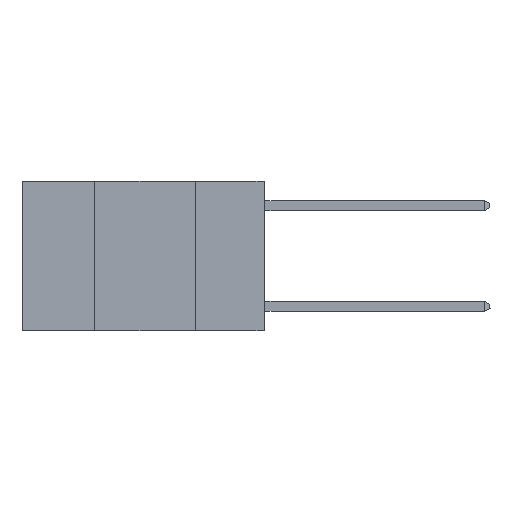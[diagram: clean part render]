
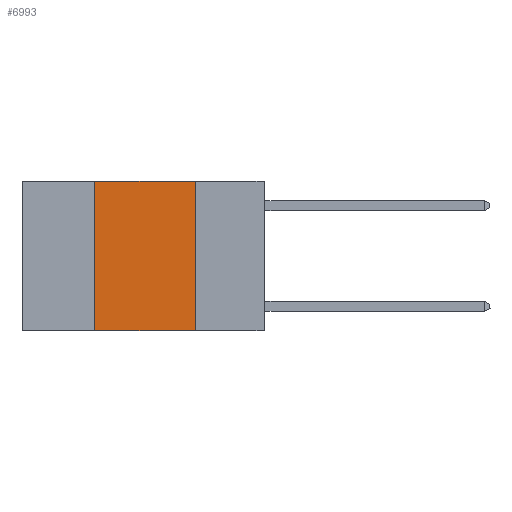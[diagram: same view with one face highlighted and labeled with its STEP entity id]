
A CAD part, left-side view. The second image highlights one B-rep face of the part: STEP entity #6993.
In plain terms, the highlighted planar face has unit normal (-1, 0, 0).
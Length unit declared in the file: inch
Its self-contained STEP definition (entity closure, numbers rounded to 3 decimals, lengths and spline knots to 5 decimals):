
#222 = LINE ( 'NONE', #16359, #4360 ) ;
#323 = CARTESIAN_POINT ( 'NONE',  ( 0., 0.6, 0. ) ) ;
#502 = EDGE_CURVE ( 'NONE', #11718, #2561, #11325, .T. ) ;
#752 = ORIENTED_EDGE ( 'NONE', *, *, #502, .T. ) ;
#1548 = VERTEX_POINT ( 'NONE', #15303 ) ;
#1932 = VECTOR ( 'NONE', #12498, 39.37008 ) ;
#2561 = VERTEX_POINT ( 'NONE', #7889 ) ;
#3376 = CARTESIAN_POINT ( 'NONE',  ( 0., 0.42, -0.37 ) ) ;
#3868 = VERTEX_POINT ( 'NONE', #14357 ) ;
#4075 = VECTOR ( 'NONE', #8578, 39.37008 ) ;
#4360 = VECTOR ( 'NONE', #13829, 39.37008 ) ;
#4531 = EDGE_CURVE ( 'NONE', #1548, #3868, #16150, .T. ) ;
#6703 = ORIENTED_EDGE ( 'NONE', *, *, #7121, .F. ) ;
#6993 = ADVANCED_FACE ( 'NONE', ( #16501 ), #15882, .F. ) ;
#7025 = CARTESIAN_POINT ( 'NONE',  ( 0., 0.6, -0.37 ) ) ;
#7121 = EDGE_CURVE ( 'NONE', #3868, #2561, #222, .T. ) ;
#7889 = CARTESIAN_POINT ( 'NONE',  ( 0., 0.17, -0.37 ) ) ;
#7894 = CARTESIAN_POINT ( 'NONE',  ( 0., 0.42, 0. ) ) ;
#8578 = DIRECTION ( 'NONE',  ( 0., -1., 0. ) ) ;
#9087 = VECTOR ( 'NONE', #9230, 39.37008 ) ;
#9230 = DIRECTION ( 'NONE',  ( 0., 0., 1. ) ) ;
#9497 = LINE ( 'NONE', #7894, #9087 ) ;
#9546 = DIRECTION ( 'NONE',  ( 0., 0., -1. ) ) ;
#9574 = AXIS2_PLACEMENT_3D ( 'NONE', #13344, #17139, #9546 ) ;
#10482 = EDGE_LOOP ( 'NONE', ( #6703, #14450, #12116, #752 ) ) ;
#11325 = LINE ( 'NONE', #7025, #4075 ) ;
#11718 = VERTEX_POINT ( 'NONE', #3376 ) ;
#11863 = EDGE_CURVE ( 'NONE', #11718, #1548, #9497, .T. ) ;
#12116 = ORIENTED_EDGE ( 'NONE', *, *, #11863, .F. ) ;
#12498 = DIRECTION ( 'NONE',  ( 0., -1., 0. ) ) ;
#13344 = CARTESIAN_POINT ( 'NONE',  ( 0., 0.6, 0. ) ) ;
#13829 = DIRECTION ( 'NONE',  ( 0., 0., -1. ) ) ;
#14357 = CARTESIAN_POINT ( 'NONE',  ( 0., 0.17, 0. ) ) ;
#14450 = ORIENTED_EDGE ( 'NONE', *, *, #4531, .F. ) ;
#15303 = CARTESIAN_POINT ( 'NONE',  ( 0., 0.42, 0. ) ) ;
#15882 = PLANE ( 'NONE',  #9574 ) ;
#16150 = LINE ( 'NONE', #323, #1932 ) ;
#16359 = CARTESIAN_POINT ( 'NONE',  ( 0., 0.17, 0. ) ) ;
#16501 = FACE_OUTER_BOUND ( 'NONE', #10482, .T. ) ;
#17139 = DIRECTION ( 'NONE',  ( 1., 0., 0. ) ) ;
